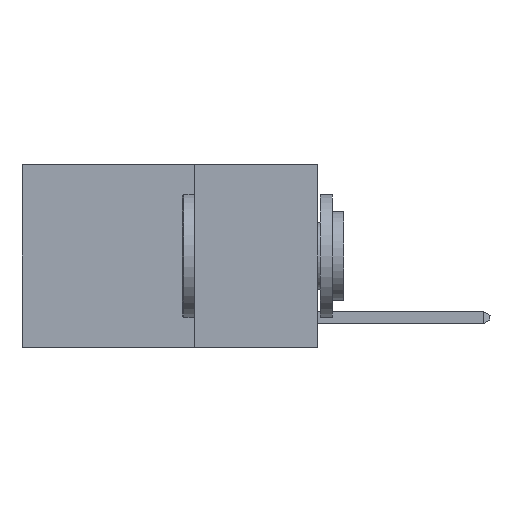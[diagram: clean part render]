
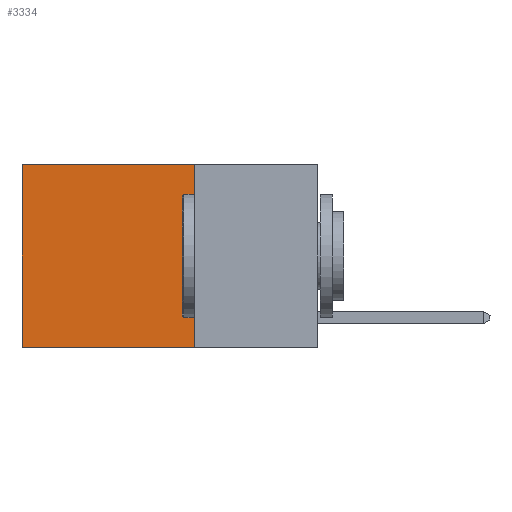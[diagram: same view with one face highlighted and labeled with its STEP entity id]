
A CAD part, left-side view. The second image highlights one B-rep face of the part: STEP entity #3334.
In plain terms, the highlighted planar face has unit normal (-1, 0, 0).
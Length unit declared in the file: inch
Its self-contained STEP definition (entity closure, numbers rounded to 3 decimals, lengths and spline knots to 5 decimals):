
#155 = CARTESIAN_POINT ( 'NONE',  ( 0.2625, 0.25, 0. ) ) ;
#965 = CARTESIAN_POINT ( 'NONE',  ( 0.2625, 0.6, -0.37 ) ) ;
#1206 = ORIENTED_EDGE ( 'NONE', *, *, #4149, .T. ) ;
#1223 = EDGE_CURVE ( 'NONE', #1869, #19395, #12313, .T. ) ;
#1230 = ORIENTED_EDGE ( 'NONE', *, *, #4939, .F. ) ;
#1264 = VECTOR ( 'NONE', #10758, 39.37008 ) ;
#1506 = EDGE_CURVE ( 'NONE', #10910, #19395, #7655, .T. ) ;
#1869 = VERTEX_POINT ( 'NONE', #7140 ) ;
#1949 = ORIENTED_EDGE ( 'NONE', *, *, #1506, .T. ) ;
#2089 = AXIS2_PLACEMENT_3D ( 'NONE', #11936, #16566, #10899 ) ;
#2729 = DIRECTION ( 'NONE',  ( 0., 1., 0. ) ) ;
#3334 = ADVANCED_FACE ( 'NONE', ( #3912 ), #10037, .F. ) ;
#3912 = FACE_OUTER_BOUND ( 'NONE', #11879, .T. ) ;
#4149 = EDGE_CURVE ( 'NONE', #7199, #10910, #13488, .T. ) ;
#4675 = CARTESIAN_POINT ( 'NONE',  ( 0.2625, 0.25, -0.37 ) ) ;
#4939 = EDGE_CURVE ( 'NONE', #7199, #1869, #19581, .T. ) ;
#7117 = CARTESIAN_POINT ( 'NONE',  ( 0.2625, 0.25, 0. ) ) ;
#7140 = CARTESIAN_POINT ( 'NONE',  ( 0.2625, 0.25, -0.37 ) ) ;
#7199 = VERTEX_POINT ( 'NONE', #155 ) ;
#7360 = CARTESIAN_POINT ( 'NONE',  ( 0.2625, 0.25, 0. ) ) ;
#7655 = LINE ( 'NONE', #16890, #1264 ) ;
#8809 = DIRECTION ( 'NONE',  ( 0., 0., -1. ) ) ;
#10037 = PLANE ( 'NONE',  #2089 ) ;
#10199 = VECTOR ( 'NONE', #15631, 39.37008 ) ;
#10758 = DIRECTION ( 'NONE',  ( 0., 0., -1. ) ) ;
#10899 = DIRECTION ( 'NONE',  ( 0., 0., -1. ) ) ;
#10910 = VERTEX_POINT ( 'NONE', #17689 ) ;
#11879 = EDGE_LOOP ( 'NONE', ( #1949, #15238, #1230, #1206 ) ) ;
#11936 = CARTESIAN_POINT ( 'NONE',  ( 0.2625, 0.25, 0. ) ) ;
#12313 = LINE ( 'NONE', #4675, #10199 ) ;
#13488 = LINE ( 'NONE', #7360, #14106 ) ;
#14106 = VECTOR ( 'NONE', #2729, 39.37008 ) ;
#15238 = ORIENTED_EDGE ( 'NONE', *, *, #1223, .F. ) ;
#15631 = DIRECTION ( 'NONE',  ( 0., 1., 0. ) ) ;
#16566 = DIRECTION ( 'NONE',  ( 1., 0., 0. ) ) ;
#16890 = CARTESIAN_POINT ( 'NONE',  ( 0.2625, 0.6, 0. ) ) ;
#17689 = CARTESIAN_POINT ( 'NONE',  ( 0.2625, 0.6, 0. ) ) ;
#18062 = VECTOR ( 'NONE', #8809, 39.37008 ) ;
#19395 = VERTEX_POINT ( 'NONE', #965 ) ;
#19581 = LINE ( 'NONE', #7117, #18062 ) ;
